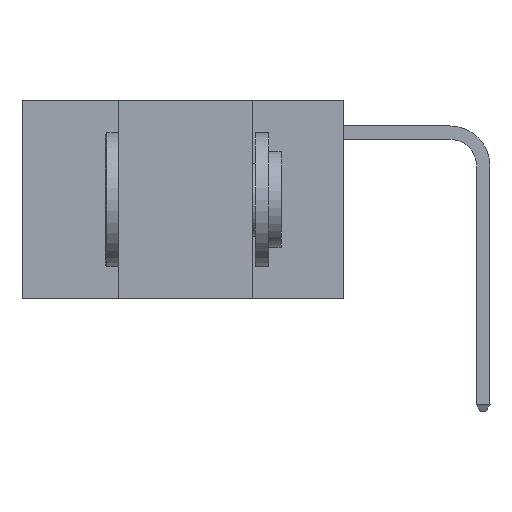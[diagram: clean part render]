
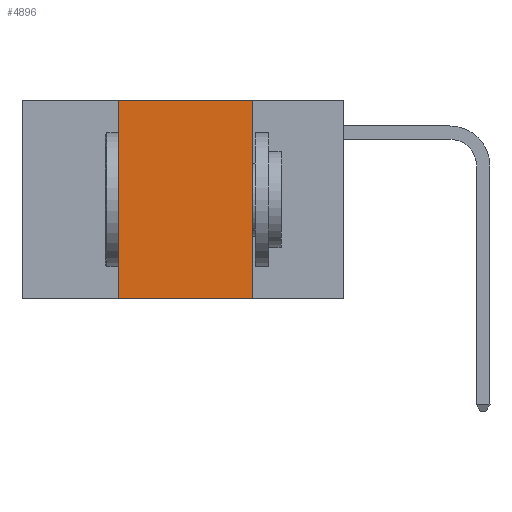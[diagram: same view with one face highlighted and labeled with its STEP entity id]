
A CAD part, left-side view. The second image highlights one B-rep face of the part: STEP entity #4896.
In plain terms, the highlighted planar face has unit normal (-1, 0, 0).
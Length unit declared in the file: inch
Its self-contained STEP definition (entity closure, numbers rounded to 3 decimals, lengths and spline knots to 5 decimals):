
#117 = ORIENTED_EDGE ( 'NONE', *, *, #6663, .F. ) ;
#644 = EDGE_CURVE ( 'NONE', #14398, #11424, #7685, .T. ) ;
#1342 = EDGE_LOOP ( 'NONE', ( #17450, #117, #5122, #12927 ) ) ;
#1418 = EDGE_CURVE ( 'NONE', #14398, #9137, #2776, .T. ) ;
#1484 = DIRECTION ( 'NONE',  ( 0., -1., 0. ) ) ;
#1486 = CARTESIAN_POINT ( 'NONE',  ( 0., 0.42, 0. ) ) ;
#1810 = DIRECTION ( 'NONE',  ( 0., 0., -1. ) ) ;
#2776 = LINE ( 'NONE', #1486, #9128 ) ;
#3970 = LINE ( 'NONE', #6896, #10091 ) ;
#4896 = ADVANCED_FACE ( 'NONE', ( #13987 ), #12435, .F. ) ;
#5122 = ORIENTED_EDGE ( 'NONE', *, *, #1418, .F. ) ;
#5189 = CARTESIAN_POINT ( 'NONE',  ( 0., 0.17, 0. ) ) ;
#5970 = CARTESIAN_POINT ( 'NONE',  ( 0., 0.17, -0.37 ) ) ;
#6228 = CARTESIAN_POINT ( 'NONE',  ( 0., 0.42, 0. ) ) ;
#6663 = EDGE_CURVE ( 'NONE', #9137, #17087, #3970, .T. ) ;
#6896 = CARTESIAN_POINT ( 'NONE',  ( 0., 0.6, 0. ) ) ;
#7685 = LINE ( 'NONE', #10767, #7724 ) ;
#7724 = VECTOR ( 'NONE', #17468, 39.37008 ) ;
#8369 = DIRECTION ( 'NONE',  ( 0., 0., 1. ) ) ;
#9128 = VECTOR ( 'NONE', #8369, 39.37008 ) ;
#9137 = VERTEX_POINT ( 'NONE', #6228 ) ;
#10091 = VECTOR ( 'NONE', #1484, 39.37008 ) ;
#10767 = CARTESIAN_POINT ( 'NONE',  ( 0., 0.6, -0.37 ) ) ;
#10898 = CARTESIAN_POINT ( 'NONE',  ( 0., 0.42, -0.37 ) ) ;
#11070 = DIRECTION ( 'NONE',  ( 1., 0., 0. ) ) ;
#11424 = VERTEX_POINT ( 'NONE', #5970 ) ;
#11785 = CARTESIAN_POINT ( 'NONE',  ( 0., 0.17, 0. ) ) ;
#12435 = PLANE ( 'NONE',  #15683 ) ;
#12865 = VECTOR ( 'NONE', #1810, 39.37008 ) ;
#12927 = ORIENTED_EDGE ( 'NONE', *, *, #644, .T. ) ;
#13615 = DIRECTION ( 'NONE',  ( 0., 0., -1. ) ) ;
#13854 = EDGE_CURVE ( 'NONE', #17087, #11424, #15890, .T. ) ;
#13987 = FACE_OUTER_BOUND ( 'NONE', #1342, .T. ) ;
#14398 = VERTEX_POINT ( 'NONE', #10898 ) ;
#15683 = AXIS2_PLACEMENT_3D ( 'NONE', #17850, #11070, #13615 ) ;
#15890 = LINE ( 'NONE', #11785, #12865 ) ;
#17087 = VERTEX_POINT ( 'NONE', #5189 ) ;
#17450 = ORIENTED_EDGE ( 'NONE', *, *, #13854, .F. ) ;
#17468 = DIRECTION ( 'NONE',  ( 0., -1., 0. ) ) ;
#17850 = CARTESIAN_POINT ( 'NONE',  ( 0., 0.6, 0. ) ) ;
